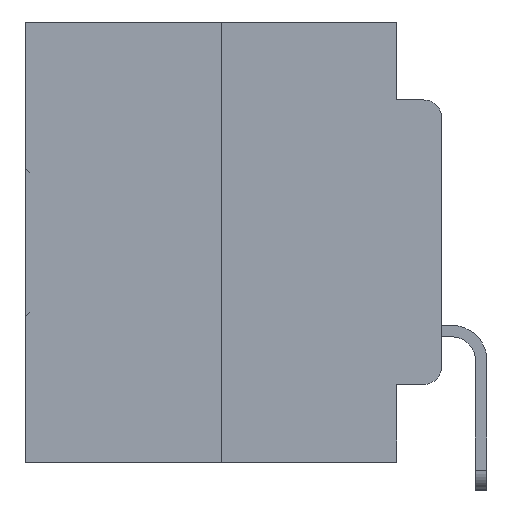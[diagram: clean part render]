
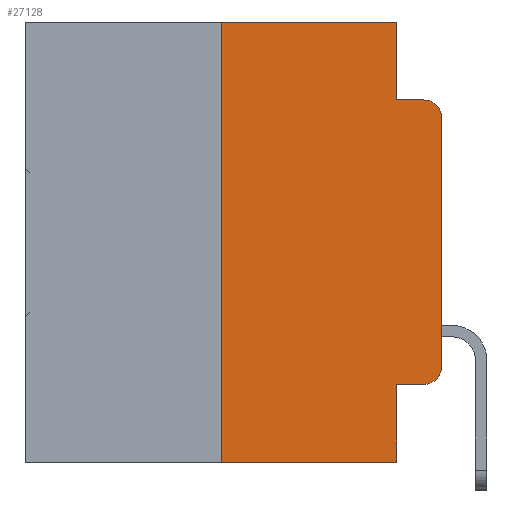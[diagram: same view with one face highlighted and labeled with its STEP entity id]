
A CAD part, left-side view. The second image highlights one B-rep face of the part: STEP entity #27128.
In plain terms, the highlighted planar face has unit normal (-1, 0, 0).
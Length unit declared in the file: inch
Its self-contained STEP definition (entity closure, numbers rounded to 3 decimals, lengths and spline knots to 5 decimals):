
#87 = VERTEX_POINT ( 'NONE', #14320 ) ;
#1002 = DIRECTION ( 'NONE',  ( 0., 0., -1. ) ) ;
#1364 = ORIENTED_EDGE ( 'NONE', *, *, #4673, .F. ) ;
#2599 = VECTOR ( 'NONE', #10003, 39.37008 ) ;
#3391 = EDGE_CURVE ( 'NONE', #13320, #4060, #23916, .T. ) ;
#3809 = VECTOR ( 'NONE', #8804, 39.37008 ) ;
#4060 = VERTEX_POINT ( 'NONE', #5869 ) ;
#4212 = ORIENTED_EDGE ( 'NONE', *, *, #19827, .F. ) ;
#4673 = EDGE_CURVE ( 'NONE', #21074, #8059, #15840, .T. ) ;
#5102 = CARTESIAN_POINT ( 'NONE',  ( 0., 0.051, 0. ) ) ;
#5130 = CARTESIAN_POINT ( 'NONE',  ( 0., 0.25, 0. ) ) ;
#5494 = AXIS2_PLACEMENT_3D ( 'NONE', #10513, #26961, #13024 ) ;
#5602 = EDGE_CURVE ( 'NONE', #17235, #4060, #26257, .T. ) ;
#5699 = LINE ( 'NONE', #16055, #30177 ) ;
#5869 = CARTESIAN_POINT ( 'NONE',  ( 0., 0.051, -0.5 ) ) ;
#6605 = VERTEX_POINT ( 'NONE', #27009 ) ;
#6619 = ORIENTED_EDGE ( 'NONE', *, *, #18259, .F. ) ;
#7033 = VERTEX_POINT ( 'NONE', #9196 ) ;
#7788 = CARTESIAN_POINT ( 'NONE',  ( 0., 0.473, -0.5 ) ) ;
#8012 = CARTESIAN_POINT ( 'NONE',  ( 0., 0.051, -0.4115 ) ) ;
#8059 = VERTEX_POINT ( 'NONE', #5102 ) ;
#8804 = DIRECTION ( 'NONE',  ( 0., -1., 0. ) ) ;
#9196 = CARTESIAN_POINT ( 'NONE',  ( 0., 0.02, -0.4115 ) ) ;
#9405 = LINE ( 'NONE', #5130, #2599 ) ;
#10003 = DIRECTION ( 'NONE',  ( 0., 0., 1. ) ) ;
#10206 = EDGE_CURVE ( 'NONE', #17235, #21074, #9405, .T. ) ;
#10468 = VECTOR ( 'NONE', #29566, 39.37008 ) ;
#10513 = CARTESIAN_POINT ( 'NONE',  ( 0., 0.473, 0. ) ) ;
#10883 = CARTESIAN_POINT ( 'NONE',  ( 0., 0.051, -0.0885 ) ) ;
#12169 = VECTOR ( 'NONE', #17380, 39.37008 ) ;
#12410 = CARTESIAN_POINT ( 'NONE',  ( 0., 0.02, -0.0885 ) ) ;
#12795 = CARTESIAN_POINT ( 'NONE',  ( 0., 0.02, -0.3915 ) ) ;
#13024 = DIRECTION ( 'NONE',  ( 0., 0., -1. ) ) ;
#13297 = AXIS2_PLACEMENT_3D ( 'NONE', #13589, #29734, #15952 ) ;
#13320 = VERTEX_POINT ( 'NONE', #8012 ) ;
#13589 = CARTESIAN_POINT ( 'NONE',  ( 0., 0.02, -0.1085 ) ) ;
#13742 = DIRECTION ( 'NONE',  ( 0., -1., 0. ) ) ;
#13816 = CARTESIAN_POINT ( 'NONE',  ( 0., 0.051, -0.4115 ) ) ;
#13937 = CIRCLE ( 'NONE', #27914, 0.02 ) ;
#14320 = CARTESIAN_POINT ( 'NONE',  ( 0., 0.051, -0.0885 ) ) ;
#15178 = ORIENTED_EDGE ( 'NONE', *, *, #26573, .T. ) ;
#15207 = DIRECTION ( 'NONE',  ( 0., 0., -1. ) ) ;
#15840 = LINE ( 'NONE', #25324, #27410 ) ;
#15952 = DIRECTION ( 'NONE',  ( 0., 0., -1. ) ) ;
#16055 = CARTESIAN_POINT ( 'NONE',  ( 0., 0.051, 0. ) ) ;
#16261 = ORIENTED_EDGE ( 'NONE', *, *, #10206, .F. ) ;
#16291 = CARTESIAN_POINT ( 'NONE',  ( 0., 0., 0. ) ) ;
#16967 = LINE ( 'NONE', #13816, #3809 ) ;
#17235 = VERTEX_POINT ( 'NONE', #22217 ) ;
#17370 = LINE ( 'NONE', #16291, #28204 ) ;
#17380 = DIRECTION ( 'NONE',  ( 0., 0., -1. ) ) ;
#17900 = VERTEX_POINT ( 'NONE', #12410 ) ;
#18259 = EDGE_CURVE ( 'NONE', #8059, #87, #5699, .T. ) ;
#18641 = DIRECTION ( 'NONE',  ( 0., 0., 1. ) ) ;
#18851 = EDGE_CURVE ( 'NONE', #7033, #6605, #13937, .T. ) ;
#19300 = CIRCLE ( 'NONE', #13297, 0.02 ) ;
#19413 = VECTOR ( 'NONE', #29054, 39.37008 ) ;
#19827 = EDGE_CURVE ( 'NONE', #87, #17900, #29153, .T. ) ;
#19879 = CARTESIAN_POINT ( 'NONE',  ( 0., 0., -0.1085 ) ) ;
#19913 = ORIENTED_EDGE ( 'NONE', *, *, #3391, .F. ) ;
#20609 = ORIENTED_EDGE ( 'NONE', *, *, #29059, .T. ) ;
#21074 = VERTEX_POINT ( 'NONE', #29752 ) ;
#21333 = ORIENTED_EDGE ( 'NONE', *, *, #27543, .T. ) ;
#21725 = EDGE_LOOP ( 'NONE', ( #20609, #21333, #4212, #6619, #1364, #16261, #29240, #19913, #15178, #27477 ) ) ;
#22217 = CARTESIAN_POINT ( 'NONE',  ( 0., 0.25, -0.5 ) ) ;
#23916 = LINE ( 'NONE', #31148, #12169 ) ;
#24574 = FACE_OUTER_BOUND ( 'NONE', #21725, .T. ) ;
#25324 = CARTESIAN_POINT ( 'NONE',  ( 0., 0.473, 0. ) ) ;
#25522 = VERTEX_POINT ( 'NONE', #19879 ) ;
#26257 = LINE ( 'NONE', #7788, #19413 ) ;
#26573 = EDGE_CURVE ( 'NONE', #13320, #7033, #16967, .T. ) ;
#26961 = DIRECTION ( 'NONE',  ( 1., 0., 0. ) ) ;
#27009 = CARTESIAN_POINT ( 'NONE',  ( 0., 0., -0.3915 ) ) ;
#27128 = ADVANCED_FACE ( 'NONE', ( #24574 ), #29142, .F. ) ;
#27410 = VECTOR ( 'NONE', #13742, 39.37008 ) ;
#27477 = ORIENTED_EDGE ( 'NONE', *, *, #18851, .T. ) ;
#27543 = EDGE_CURVE ( 'NONE', #25522, #17900, #19300, .T. ) ;
#27914 = AXIS2_PLACEMENT_3D ( 'NONE', #12795, #29024, #15207 ) ;
#28204 = VECTOR ( 'NONE', #18641, 39.37008 ) ;
#29024 = DIRECTION ( 'NONE',  ( -1., 0., 0. ) ) ;
#29054 = DIRECTION ( 'NONE',  ( 0., -1., 0. ) ) ;
#29059 = EDGE_CURVE ( 'NONE', #6605, #25522, #17370, .T. ) ;
#29142 = PLANE ( 'NONE',  #5494 ) ;
#29153 = LINE ( 'NONE', #10883, #10468 ) ;
#29240 = ORIENTED_EDGE ( 'NONE', *, *, #5602, .T. ) ;
#29566 = DIRECTION ( 'NONE',  ( 0., -1., 0. ) ) ;
#29734 = DIRECTION ( 'NONE',  ( -1., 0., 0. ) ) ;
#29752 = CARTESIAN_POINT ( 'NONE',  ( 0., 0.25, 0. ) ) ;
#30177 = VECTOR ( 'NONE', #1002, 39.37008 ) ;
#31148 = CARTESIAN_POINT ( 'NONE',  ( 0., 0.051, 0. ) ) ;
